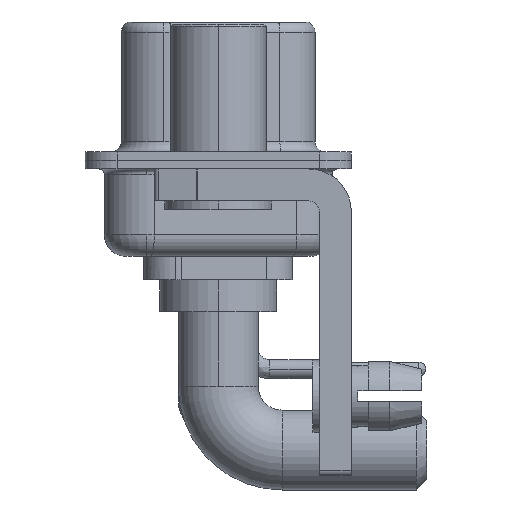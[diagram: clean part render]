
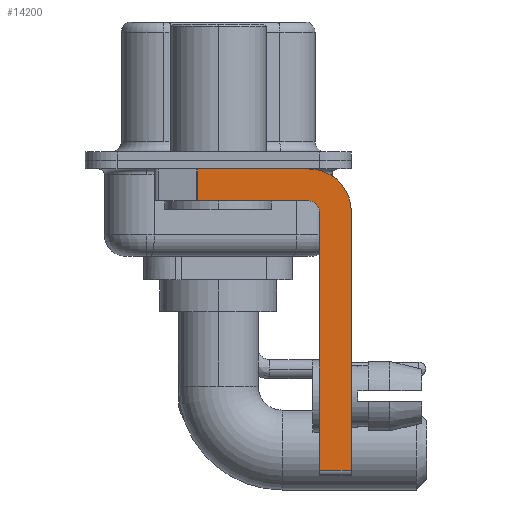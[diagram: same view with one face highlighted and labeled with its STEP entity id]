
A CAD part, left-side view. The second image highlights one B-rep face of the part: STEP entity #14200.
In plain terms, the highlighted planar face has unit normal (-1, 0, 0).
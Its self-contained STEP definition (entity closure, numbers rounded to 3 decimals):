
#63 = EDGE_CURVE ( 'NONE', #12698, #4013, #5643, .T. ) ;
#198 = ORIENTED_EDGE ( 'NONE', *, *, #19880, .F. ) ;
#1141 = CARTESIAN_POINT ( 'NONE',  ( -2.9, -4.25, -1.9 ) ) ;
#2123 = AXIS2_PLACEMENT_3D ( 'NONE', #25339, #6547, #4596 ) ;
#2714 = AXIS2_PLACEMENT_3D ( 'NONE', #22980, #4558, #23520 ) ;
#3140 = CIRCLE ( 'NONE', #2714, 2. ) ;
#4013 = VERTEX_POINT ( 'NONE', #11597 ) ;
#4342 = FACE_OUTER_BOUND ( 'NONE', #4635, .T. ) ;
#4558 = DIRECTION ( 'NONE',  ( 1., 0., 0. ) ) ;
#4596 = DIRECTION ( 'NONE',  ( 0., 0., -1. ) ) ;
#4635 = EDGE_LOOP ( 'NONE', ( #8726, #15344, #20245, #16273, #25240, #9527, #12183, #198 ) ) ;
#5643 = LINE ( 'NONE', #9918, #8248 ) ;
#5656 = DIRECTION ( 'NONE',  ( 0., 0., -1. ) ) ;
#5909 = EDGE_CURVE ( 'NONE', #16473, #9590, #14204, .T. ) ;
#6195 = DIRECTION ( 'NONE',  ( 0., 0., 1. ) ) ;
#6547 = DIRECTION ( 'NONE',  ( 1., 0., 0. ) ) ;
#6908 = CARTESIAN_POINT ( 'NONE',  ( -2.9, 0.978, -1.9 ) ) ;
#7039 = LINE ( 'NONE', #13092, #23467 ) ;
#7044 = DIRECTION ( 'NONE',  ( 0., 1., 0. ) ) ;
#7067 = EDGE_CURVE ( 'NONE', #12698, #9590, #26402, .T. ) ;
#7740 = CARTESIAN_POINT ( 'NONE',  ( -2.9, -6.25, -2.4 ) ) ;
#7929 = VERTEX_POINT ( 'NONE', #24517 ) ;
#8172 = LINE ( 'NONE', #14626, #24680 ) ;
#8248 = VECTOR ( 'NONE', #26658, 1000. ) ;
#8399 = DIRECTION ( 'NONE',  ( -1., 0., 0. ) ) ;
#8532 = CARTESIAN_POINT ( 'NONE',  ( -2.9, -4.25, -2.4 ) ) ;
#8726 = ORIENTED_EDGE ( 'NONE', *, *, #26660, .F. ) ;
#9515 = LINE ( 'NONE', #1141, #18054 ) ;
#9527 = ORIENTED_EDGE ( 'NONE', *, *, #7067, .T. ) ;
#9590 = VERTEX_POINT ( 'NONE', #15724 ) ;
#9918 = CARTESIAN_POINT ( 'NONE',  ( -2.9, -4.75, -14.8 ) ) ;
#10082 = DIRECTION ( 'NONE',  ( 0., 0., -1. ) ) ;
#10718 = CARTESIAN_POINT ( 'NONE',  ( -2.9, 0.978, -0.4 ) ) ;
#11597 = CARTESIAN_POINT ( 'NONE',  ( -2.9, -4.75, -2.4 ) ) ;
#11629 = VERTEX_POINT ( 'NONE', #10718 ) ;
#12183 = ORIENTED_EDGE ( 'NONE', *, *, #5909, .F. ) ;
#12698 = VERTEX_POINT ( 'NONE', #25858 ) ;
#13092 = CARTESIAN_POINT ( 'NONE',  ( -2.9, 3., -0.4 ) ) ;
#13342 = VECTOR ( 'NONE', #23810, 1000. ) ;
#13542 = CARTESIAN_POINT ( 'NONE',  ( -2.9, -4.25, -14.55 ) ) ;
#14200 = ADVANCED_FACE ( 'NONE', ( #4342 ), #16998, .F. ) ;
#14204 = LINE ( 'NONE', #7740, #18716 ) ;
#14626 = CARTESIAN_POINT ( 'NONE',  ( -2.9, 0.978, -1.9 ) ) ;
#15344 = ORIENTED_EDGE ( 'NONE', *, *, #24906, .T. ) ;
#15724 = CARTESIAN_POINT ( 'NONE',  ( -2.9, -6.25, -14.55 ) ) ;
#16273 = ORIENTED_EDGE ( 'NONE', *, *, #22156, .F. ) ;
#16335 = CARTESIAN_POINT ( 'NONE',  ( -2.9, -4.25, -1.9 ) ) ;
#16473 = VERTEX_POINT ( 'NONE', #22180 ) ;
#16998 = PLANE ( 'NONE',  #2123 ) ;
#18054 = VECTOR ( 'NONE', #7044, 1000. ) ;
#18716 = VECTOR ( 'NONE', #5656, 1000. ) ;
#19391 = CIRCLE ( 'NONE', #26820, 0.5 ) ;
#19880 = EDGE_CURVE ( 'NONE', #7929, #16473, #3140, .T. ) ;
#19924 = EDGE_CURVE ( 'NONE', #25813, #21877, #9515, .T. ) ;
#20245 = ORIENTED_EDGE ( 'NONE', *, *, #19924, .F. ) ;
#21877 = VERTEX_POINT ( 'NONE', #6908 ) ;
#22156 = EDGE_CURVE ( 'NONE', #4013, #25813, #19391, .T. ) ;
#22180 = CARTESIAN_POINT ( 'NONE',  ( -2.9, -6.25, -2.4 ) ) ;
#22980 = CARTESIAN_POINT ( 'NONE',  ( -2.9, -4.25, -2.4 ) ) ;
#23467 = VECTOR ( 'NONE', #23772, 1000. ) ;
#23520 = DIRECTION ( 'NONE',  ( 0., 0., -1. ) ) ;
#23772 = DIRECTION ( 'NONE',  ( 0., -1., 0. ) ) ;
#23810 = DIRECTION ( 'NONE',  ( 0., -1., 0. ) ) ;
#24517 = CARTESIAN_POINT ( 'NONE',  ( -2.9, -4.25, -0.4 ) ) ;
#24680 = VECTOR ( 'NONE', #10082, 1000. ) ;
#24906 = EDGE_CURVE ( 'NONE', #11629, #21877, #8172, .T. ) ;
#25240 = ORIENTED_EDGE ( 'NONE', *, *, #63, .F. ) ;
#25339 = CARTESIAN_POINT ( 'NONE',  ( -2.9, -4.25, -2.4 ) ) ;
#25813 = VERTEX_POINT ( 'NONE', #16335 ) ;
#25858 = CARTESIAN_POINT ( 'NONE',  ( -2.9, -4.75, -14.55 ) ) ;
#26402 = LINE ( 'NONE', #13542, #13342 ) ;
#26658 = DIRECTION ( 'NONE',  ( 0., 0., 1. ) ) ;
#26660 = EDGE_CURVE ( 'NONE', #11629, #7929, #7039, .T. ) ;
#26820 = AXIS2_PLACEMENT_3D ( 'NONE', #8532, #8399, #6195 ) ;
